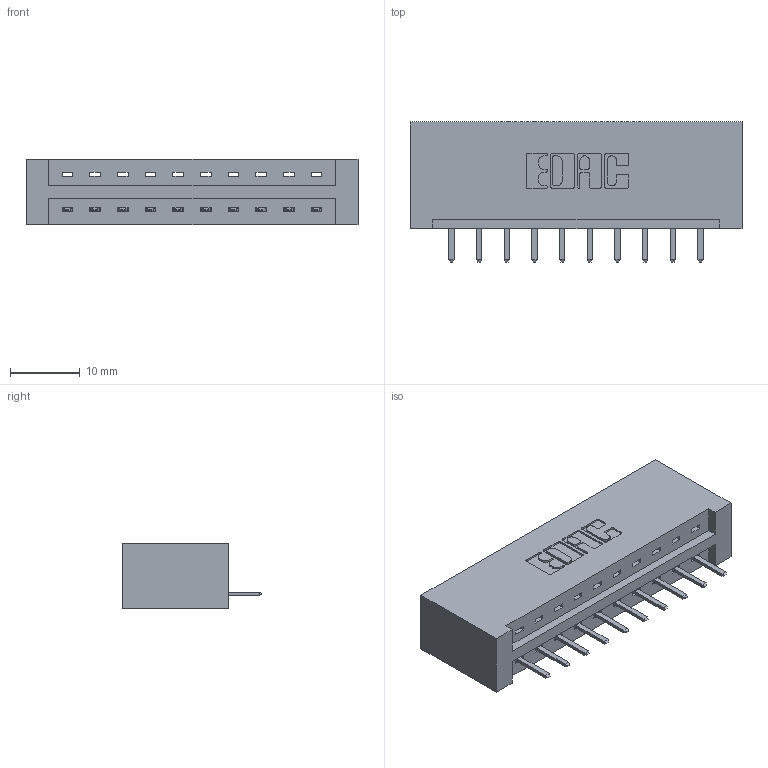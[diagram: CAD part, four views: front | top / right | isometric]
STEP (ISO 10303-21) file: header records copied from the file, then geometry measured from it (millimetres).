
FILE_DESCRIPTION (( 'STEP AP203' ), '1' );
FILE_NAME ('387-010-520-101.STEP', '2018-09-10T06:25:49', ( '' ), ( '' ), 'SwSTEP 2.0', 'SolidWorks 2016', '' );
FILE_SCHEMA (( 'CONFIG_CONTROL_DESIGN' ));
Length unit declared in the file: inch
Products named in the file (3): 337 Part_No Mounting Lugs; 345-292-001_345-293-120; 387-010-520-101
Assembly tree (11 placements, depth 2):
  387-010-520-101
    337 Part_No Mounting Lugs
    345-292-001_345-293-120  x10
Bounding box: 47.5 x 20.02 x 9.4 mm (x, y, z)
Volume: 5246.1 mm3; surface area: 5121.4 mm2
Topology: 11 solids, 11 shells, 766 faces, 2247 edges, 1470 vertices
Faces by surface type: plane 546, cylinder 220
Entity records: 11409 total; most frequent: CARTESIAN_POINT 2004, ORIENTED_EDGE 1938, DIRECTION 1733, EDGE_CURVE 969, LINE 845, VECTOR 845, VERTEX_POINT 642, AXIS2_PLACEMENT_3D 444
